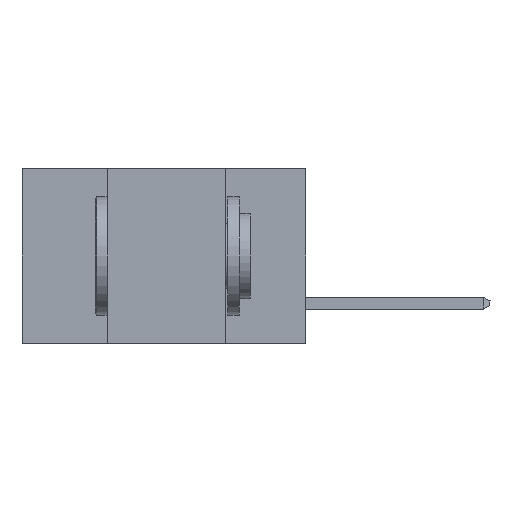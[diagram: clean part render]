
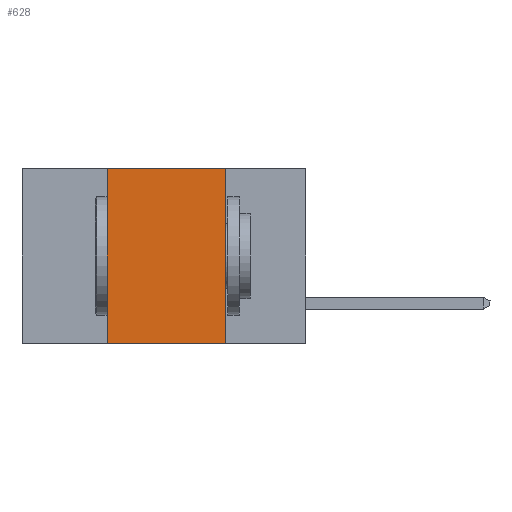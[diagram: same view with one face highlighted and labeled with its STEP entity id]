
A CAD part, left-side view. The second image highlights one B-rep face of the part: STEP entity #628.
In plain terms, the highlighted planar face has unit normal (-1, 0, 0).
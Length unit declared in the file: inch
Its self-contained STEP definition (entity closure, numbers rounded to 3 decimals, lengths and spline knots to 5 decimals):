
#628 = ADVANCED_FACE ( 'NONE', ( #1257 ), #21871, .F. ) ;
#697 = DIRECTION ( 'NONE',  ( 0., -1., 0. ) ) ;
#1142 = DIRECTION ( 'NONE',  ( 1., 0., 0. ) ) ;
#1257 = FACE_OUTER_BOUND ( 'NONE', #21072, .T. ) ;
#1573 = VERTEX_POINT ( 'NONE', #19995 ) ;
#2355 = LINE ( 'NONE', #17720, #8240 ) ;
#4849 = EDGE_CURVE ( 'NONE', #7829, #6283, #19725, .T. ) ;
#4970 = EDGE_CURVE ( 'NONE', #1573, #10347, #11961, .T. ) ;
#5073 = CARTESIAN_POINT ( 'NONE',  ( 0., 0.6, 0. ) ) ;
#5595 = ORIENTED_EDGE ( 'NONE', *, *, #4970, .F. ) ;
#5920 = DIRECTION ( 'NONE',  ( 0., 0., 1. ) ) ;
#6283 = VERTEX_POINT ( 'NONE', #9825 ) ;
#6599 = VECTOR ( 'NONE', #22241, 39.37008 ) ;
#6724 = CARTESIAN_POINT ( 'NONE',  ( 0., 0.42, -0.37 ) ) ;
#7352 = ORIENTED_EDGE ( 'NONE', *, *, #22391, .F. ) ;
#7603 = CARTESIAN_POINT ( 'NONE',  ( 0., 0.6, -0.37 ) ) ;
#7829 = VERTEX_POINT ( 'NONE', #6724 ) ;
#8240 = VECTOR ( 'NONE', #5920, 39.37008 ) ;
#9103 = ORIENTED_EDGE ( 'NONE', *, *, #4849, .T. ) ;
#9825 = CARTESIAN_POINT ( 'NONE',  ( 0., 0.17, -0.37 ) ) ;
#9841 = AXIS2_PLACEMENT_3D ( 'NONE', #16852, #1142, #13196 ) ;
#9868 = CARTESIAN_POINT ( 'NONE',  ( 0., 0.17, 0. ) ) ;
#10347 = VERTEX_POINT ( 'NONE', #9868 ) ;
#10568 = CARTESIAN_POINT ( 'NONE',  ( 0., 0.17, -0.37 ) ) ;
#11961 = LINE ( 'NONE', #5073, #6599 ) ;
#12105 = EDGE_CURVE ( 'NONE', #7829, #1573, #2355, .T. ) ;
#12457 = VECTOR ( 'NONE', #697, 39.37008 ) ;
#13196 = DIRECTION ( 'NONE',  ( 0., 0., -1. ) ) ;
#15376 = ORIENTED_EDGE ( 'NONE', *, *, #12105, .F. ) ;
#15948 = DIRECTION ( 'NONE',  ( 0., 0., -1. ) ) ;
#16852 = CARTESIAN_POINT ( 'NONE',  ( 0., 0.6, 0. ) ) ;
#17650 = LINE ( 'NONE', #10568, #18112 ) ;
#17720 = CARTESIAN_POINT ( 'NONE',  ( 0., 0.42, -0.37 ) ) ;
#18112 = VECTOR ( 'NONE', #15948, 39.37008 ) ;
#19725 = LINE ( 'NONE', #7603, #12457 ) ;
#19995 = CARTESIAN_POINT ( 'NONE',  ( 0., 0.42, 0. ) ) ;
#21072 = EDGE_LOOP ( 'NONE', ( #7352, #5595, #15376, #9103 ) ) ;
#21871 = PLANE ( 'NONE',  #9841 ) ;
#22241 = DIRECTION ( 'NONE',  ( 0., -1., 0. ) ) ;
#22391 = EDGE_CURVE ( 'NONE', #10347, #6283, #17650, .T. ) ;
